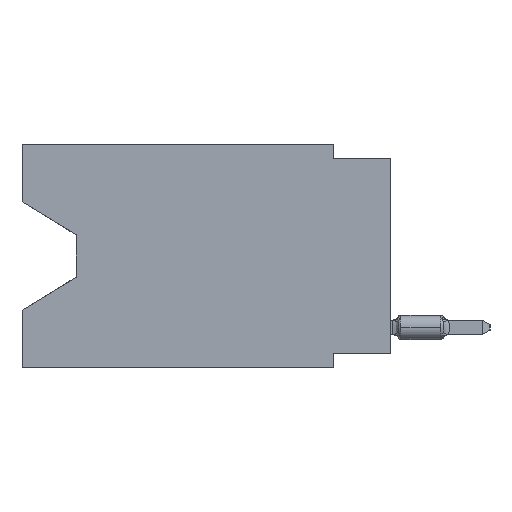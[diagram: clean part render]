
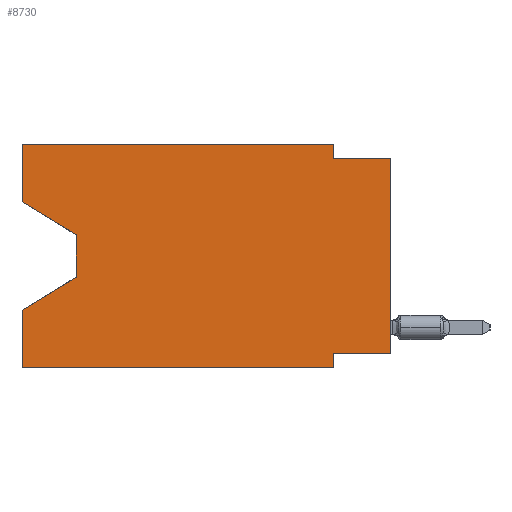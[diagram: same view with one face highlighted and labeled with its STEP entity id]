
A CAD part, left-side view. The second image highlights one B-rep face of the part: STEP entity #8730.
In plain terms, the highlighted planar face has unit normal (-1, 0, 0).
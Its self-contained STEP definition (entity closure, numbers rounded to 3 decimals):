
#492 = EDGE_CURVE ( 'NONE', #7301, #23610, #28197, .T. ) ;
#1053 = VERTEX_POINT ( 'NONE', #73250 ) ;
#1415 = LINE ( 'NONE', #74889, #37319 ) ;
#2511 = EDGE_CURVE ( 'NONE', #1053, #21171, #1415, .T. ) ;
#3797 = CARTESIAN_POINT ( 'NONE',  ( 0., 16.383, -7.36 ) ) ;
#4188 = ORIENTED_EDGE ( 'NONE', *, *, #42199, .F. ) ;
#4303 = LINE ( 'NONE', #41204, #12904 ) ;
#5520 = CARTESIAN_POINT ( 'NONE',  ( 0., 2.54, -9.906 ) ) ;
#7301 = VERTEX_POINT ( 'NONE', #76486 ) ;
#7810 = ORIENTED_EDGE ( 'NONE', *, *, #492, .F. ) ;
#7816 = VECTOR ( 'NONE', #75262, 1000. ) ;
#8157 = ORIENTED_EDGE ( 'NONE', *, *, #23309, .F. ) ;
#8730 = ADVANCED_FACE ( 'NONE', ( #68112 ), #12914, .F. ) ;
#8894 = CARTESIAN_POINT ( 'NONE',  ( 0., 16.383, 0. ) ) ;
#12430 = DIRECTION ( 'NONE',  ( 0., 0., 1. ) ) ;
#12904 = VECTOR ( 'NONE', #28523, 1000. ) ;
#12914 = PLANE ( 'NONE',  #40382 ) ;
#12939 = DIRECTION ( 'NONE',  ( 0., -0.855, -0.519 ) ) ;
#12956 = LINE ( 'NONE', #72169, #42142 ) ;
#13111 = VERTEX_POINT ( 'NONE', #3797 ) ;
#13208 = CARTESIAN_POINT ( 'NONE',  ( 0., 0., 0. ) ) ;
#13686 = CARTESIAN_POINT ( 'NONE',  ( 0., 16.383, 0. ) ) ;
#13822 = DIRECTION ( 'NONE',  ( 0., 0., 1. ) ) ;
#13987 = LINE ( 'NONE', #13208, #19892 ) ;
#14644 = VERTEX_POINT ( 'NONE', #59223 ) ;
#15866 = CARTESIAN_POINT ( 'NONE',  ( 0., 16.383, -9.906 ) ) ;
#16066 = EDGE_CURVE ( 'NONE', #70121, #23610, #26613, .T. ) ;
#16668 = LINE ( 'NONE', #53188, #19990 ) ;
#19258 = LINE ( 'NONE', #8894, #70788 ) ;
#19331 = EDGE_LOOP ( 'NONE', ( #23589, #65835, #20509, #50681, #78550, #7810, #46055, #25677, #54015, #41169, #8157, #4188 ) ) ;
#19892 = VECTOR ( 'NONE', #12430, 1000. ) ;
#19990 = VECTOR ( 'NONE', #52781, 1000. ) ;
#20509 = ORIENTED_EDGE ( 'NONE', *, *, #36770, .T. ) ;
#20893 = VERTEX_POINT ( 'NONE', #49558 ) ;
#20956 = EDGE_CURVE ( 'NONE', #70121, #13111, #61479, .T. ) ;
#21171 = VERTEX_POINT ( 'NONE', #32334 ) ;
#23309 = EDGE_CURVE ( 'NONE', #30994, #20893, #12956, .T. ) ;
#23589 = ORIENTED_EDGE ( 'NONE', *, *, #2511, .T. ) ;
#23610 = VERTEX_POINT ( 'NONE', #46647 ) ;
#24543 = CARTESIAN_POINT ( 'NONE',  ( 0., 16.383, -9.906 ) ) ;
#24606 = DIRECTION ( 'NONE',  ( 0., 1., 0. ) ) ;
#25154 = VECTOR ( 'NONE', #13822, 1000. ) ;
#25409 = CARTESIAN_POINT ( 'NONE',  ( 0., 0., -9.271 ) ) ;
#25677 = ORIENTED_EDGE ( 'NONE', *, *, #35746, .T. ) ;
#26114 = EDGE_CURVE ( 'NONE', #31193, #7301, #49615, .T. ) ;
#26213 = DIRECTION ( 'NONE',  ( 0., -1., 0. ) ) ;
#26613 = LINE ( 'NONE', #15866, #57697 ) ;
#28197 = LINE ( 'NONE', #5520, #49955 ) ;
#28523 = DIRECTION ( 'NONE',  ( 0., 0., -1. ) ) ;
#30994 = VERTEX_POINT ( 'NONE', #37269 ) ;
#31193 = VERTEX_POINT ( 'NONE', #66210 ) ;
#31928 = CARTESIAN_POINT ( 'NONE',  ( 0., 13.97, -5.893 ) ) ;
#32334 = CARTESIAN_POINT ( 'NONE',  ( 0., 13.97, -4.013 ) ) ;
#35746 = EDGE_CURVE ( 'NONE', #31193, #49602, #13987, .T. ) ;
#36770 = EDGE_CURVE ( 'NONE', #14644, #13111, #48231, .T. ) ;
#37269 = CARTESIAN_POINT ( 'NONE',  ( 0., 16.383, 0. ) ) ;
#37319 = VECTOR ( 'NONE', #12939, 1000. ) ;
#40382 = AXIS2_PLACEMENT_3D ( 'NONE', #13686, #54991, #62145 ) ;
#41169 = ORIENTED_EDGE ( 'NONE', *, *, #46338, .F. ) ;
#41204 = CARTESIAN_POINT ( 'NONE',  ( 0., 13.97, -4.013 ) ) ;
#42142 = VECTOR ( 'NONE', #61396, 1000. ) ;
#42199 = EDGE_CURVE ( 'NONE', #1053, #30994, #19258, .T. ) ;
#46055 = ORIENTED_EDGE ( 'NONE', *, *, #26114, .F. ) ;
#46338 = EDGE_CURVE ( 'NONE', #20893, #63201, #62173, .T. ) ;
#46647 = CARTESIAN_POINT ( 'NONE',  ( 0., 2.54, -9.906 ) ) ;
#48231 = LINE ( 'NONE', #31928, #59304 ) ;
#49558 = CARTESIAN_POINT ( 'NONE',  ( 0., 2.54, 0. ) ) ;
#49602 = VERTEX_POINT ( 'NONE', #66204 ) ;
#49615 = LINE ( 'NONE', #25409, #61373 ) ;
#49955 = VECTOR ( 'NONE', #59557, 1000. ) ;
#50681 = ORIENTED_EDGE ( 'NONE', *, *, #20956, .F. ) ;
#52781 = DIRECTION ( 'NONE',  ( 0., -1., 0. ) ) ;
#53188 = CARTESIAN_POINT ( 'NONE',  ( 0., 0., -0.635 ) ) ;
#54015 = ORIENTED_EDGE ( 'NONE', *, *, #71752, .F. ) ;
#54991 = DIRECTION ( 'NONE',  ( 1., 0., 0. ) ) ;
#55781 = DIRECTION ( 'NONE',  ( 0., 0., 1. ) ) ;
#56985 = CARTESIAN_POINT ( 'NONE',  ( 0., 2.54, 0. ) ) ;
#57491 = EDGE_CURVE ( 'NONE', #21171, #14644, #4303, .T. ) ;
#57697 = VECTOR ( 'NONE', #26213, 1000. ) ;
#59223 = CARTESIAN_POINT ( 'NONE',  ( 0., 13.97, -5.893 ) ) ;
#59304 = VECTOR ( 'NONE', #73666, 1000. ) ;
#59557 = DIRECTION ( 'NONE',  ( 0., 0., -1. ) ) ;
#61373 = VECTOR ( 'NONE', #24606, 1000. ) ;
#61396 = DIRECTION ( 'NONE',  ( 0., -1., 0. ) ) ;
#61479 = LINE ( 'NONE', #73024, #25154 ) ;
#62145 = DIRECTION ( 'NONE',  ( 0., 0., -1. ) ) ;
#62173 = LINE ( 'NONE', #56985, #7816 ) ;
#63201 = VERTEX_POINT ( 'NONE', #71673 ) ;
#65835 = ORIENTED_EDGE ( 'NONE', *, *, #57491, .T. ) ;
#66204 = CARTESIAN_POINT ( 'NONE',  ( 0., 0., -0.635 ) ) ;
#66210 = CARTESIAN_POINT ( 'NONE',  ( 0., 0., -9.271 ) ) ;
#68112 = FACE_OUTER_BOUND ( 'NONE', #19331, .T. ) ;
#70121 = VERTEX_POINT ( 'NONE', #24543 ) ;
#70788 = VECTOR ( 'NONE', #55781, 1000. ) ;
#71673 = CARTESIAN_POINT ( 'NONE',  ( 0., 2.54, -0.635 ) ) ;
#71752 = EDGE_CURVE ( 'NONE', #63201, #49602, #16668, .T. ) ;
#72169 = CARTESIAN_POINT ( 'NONE',  ( 0., 16.383, 0. ) ) ;
#73024 = CARTESIAN_POINT ( 'NONE',  ( 0., 16.383, 0. ) ) ;
#73250 = CARTESIAN_POINT ( 'NONE',  ( 0., 16.383, -2.546 ) ) ;
#73666 = DIRECTION ( 'NONE',  ( 0., 0.855, -0.519 ) ) ;
#74889 = CARTESIAN_POINT ( 'NONE',  ( 0., 16.383, -2.546 ) ) ;
#75262 = DIRECTION ( 'NONE',  ( 0., 0., -1. ) ) ;
#76486 = CARTESIAN_POINT ( 'NONE',  ( 0., 2.54, -9.271 ) ) ;
#78550 = ORIENTED_EDGE ( 'NONE', *, *, #16066, .T. ) ;
